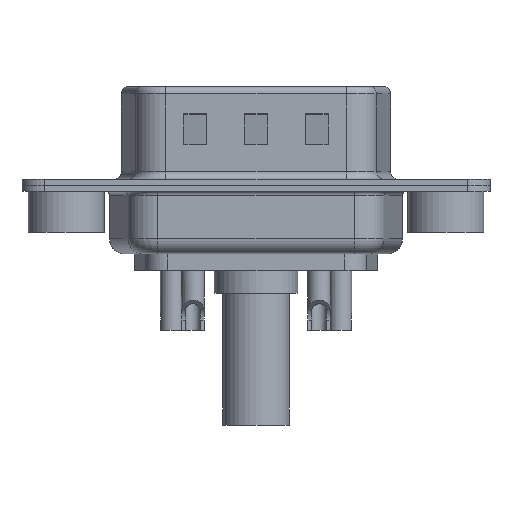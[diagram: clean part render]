
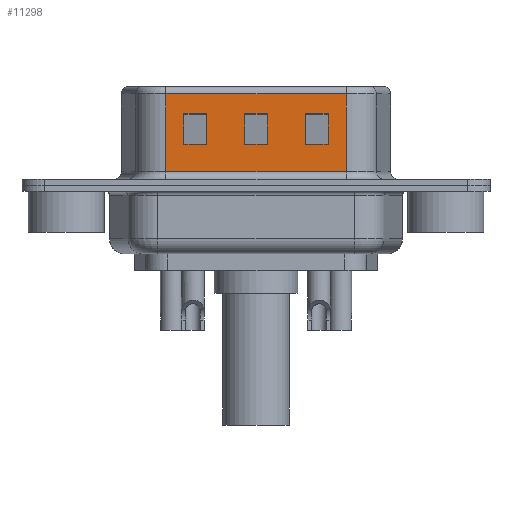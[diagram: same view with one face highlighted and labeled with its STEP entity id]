
A CAD part, front view. The second image highlights one B-rep face of the part: STEP entity #11298.
In plain terms, the highlighted planar face has unit normal (0, -1, 0).
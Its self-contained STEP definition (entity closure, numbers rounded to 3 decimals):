
#24 = VECTOR ( 'NONE', #2627, 1000. ) ;
#166 = DIRECTION ( 'NONE',  ( 0., 0., 1. ) ) ;
#189 = LINE ( 'NONE', #15808, #4331 ) ;
#196 = DIRECTION ( 'NONE',  ( -1., 0., 0. ) ) ;
#647 = CARTESIAN_POINT ( 'NONE',  ( 18.45, -4.58, 6.02 ) ) ;
#765 = EDGE_LOOP ( 'NONE', ( #6442, #6425, #10192, #7241 ) ) ;
#857 = EDGE_CURVE ( 'NONE', #8389, #2195, #1545, .T. ) ;
#917 = VECTOR ( 'NONE', #13307, 1000. ) ;
#921 = LINE ( 'NONE', #5313, #24 ) ;
#1360 = CARTESIAN_POINT ( 'NONE',  ( 15.75, -4.58, 2.705 ) ) ;
#1391 = ORIENTED_EDGE ( 'NONE', *, *, #1806, .T. ) ;
#1420 = LINE ( 'NONE', #13217, #4685 ) ;
#1493 = VECTOR ( 'NONE', #16362, 1000. ) ;
#1545 = LINE ( 'NONE', #11273, #8769 ) ;
#1702 = ORIENTED_EDGE ( 'NONE', *, *, #4582, .T. ) ;
#1806 = EDGE_CURVE ( 'NONE', #4590, #8389, #2220, .T. ) ;
#1848 = VERTEX_POINT ( 'NONE', #1360 ) ;
#1966 = CARTESIAN_POINT ( 'NONE',  ( 7.75, -4.58, 4.705 ) ) ;
#2132 = ORIENTED_EDGE ( 'NONE', *, *, #857, .T. ) ;
#2195 = VERTEX_POINT ( 'NONE', #5298 ) ;
#2220 = LINE ( 'NONE', #15970, #5825 ) ;
#2395 = ORIENTED_EDGE ( 'NONE', *, *, #9380, .T. ) ;
#2528 = DIRECTION ( 'NONE',  ( 0., 0., -1. ) ) ;
#2570 = ORIENTED_EDGE ( 'NONE', *, *, #5812, .T. ) ;
#2623 = LINE ( 'NONE', #16500, #16388 ) ;
#2627 = DIRECTION ( 'NONE',  ( -1., 0., 0. ) ) ;
#2742 = EDGE_CURVE ( 'NONE', #15333, #4590, #13022, .T. ) ;
#2941 = CARTESIAN_POINT ( 'NONE',  ( 18.45, -4.58, 6.52 ) ) ;
#3029 = VERTEX_POINT ( 'NONE', #647 ) ;
#3149 = EDGE_LOOP ( 'NONE', ( #13608, #2395, #9383, #2570 ) ) ;
#3228 = DIRECTION ( 'NONE',  ( -1., 0., 0. ) ) ;
#3500 = CARTESIAN_POINT ( 'NONE',  ( 14.45, -4.58, 2.705 ) ) ;
#3504 = DIRECTION ( 'NONE',  ( 0., 0., -1. ) ) ;
#3507 = VERTEX_POINT ( 'NONE', #7086 ) ;
#3559 = LINE ( 'NONE', #10552, #7119 ) ;
#3588 = VERTEX_POINT ( 'NONE', #13491 ) ;
#3820 = CARTESIAN_POINT ( 'NONE',  ( 9.25, -4.58, 2.705 ) ) ;
#3976 = DIRECTION ( 'NONE',  ( 1., 0., 0. ) ) ;
#4067 = DIRECTION ( 'NONE',  ( 0., 0., -1. ) ) ;
#4071 = DIRECTION ( 'NONE',  ( 0., 0., 1. ) ) ;
#4331 = VECTOR ( 'NONE', #16017, 1000. ) ;
#4582 = EDGE_CURVE ( 'NONE', #2195, #15333, #6016, .T. ) ;
#4590 = VERTEX_POINT ( 'NONE', #11797 ) ;
#4685 = VECTOR ( 'NONE', #3976, 1000. ) ;
#4841 = CARTESIAN_POINT ( 'NONE',  ( 17.25, -4.58, 2.705 ) ) ;
#4879 = CARTESIAN_POINT ( 'NONE',  ( 6.55, -4.58, 6.52 ) ) ;
#4881 = ORIENTED_EDGE ( 'NONE', *, *, #17098, .T. ) ;
#4919 = EDGE_CURVE ( 'NONE', #13281, #14281, #2623, .T. ) ;
#5298 = CARTESIAN_POINT ( 'NONE',  ( 9.25, -4.58, 4.705 ) ) ;
#5313 = CARTESIAN_POINT ( 'NONE',  ( 22.45, -4.58, 2.705 ) ) ;
#5441 = CARTESIAN_POINT ( 'NONE',  ( 18.45, -4.58, 4.705 ) ) ;
#5642 = CARTESIAN_POINT ( 'NONE',  ( 18.45, -4.58, 0.9 ) ) ;
#5812 = EDGE_CURVE ( 'NONE', #3507, #8795, #189, .T. ) ;
#5825 = VECTOR ( 'NONE', #12913, 1000. ) ;
#6016 = LINE ( 'NONE', #12508, #13404 ) ;
#6020 = LINE ( 'NONE', #7359, #12657 ) ;
#6072 = FACE_BOUND ( 'NONE', #15470, .T. ) ;
#6241 = ORIENTED_EDGE ( 'NONE', *, *, #13717, .T. ) ;
#6324 = ORIENTED_EDGE ( 'NONE', *, *, #15402, .T. ) ;
#6345 = EDGE_CURVE ( 'NONE', #3029, #16842, #8722, .T. ) ;
#6425 = ORIENTED_EDGE ( 'NONE', *, *, #6345, .T. ) ;
#6442 = ORIENTED_EDGE ( 'NONE', *, *, #9281, .F. ) ;
#6564 = CARTESIAN_POINT ( 'NONE',  ( 11.75, -4.58, 4.705 ) ) ;
#6698 = CARTESIAN_POINT ( 'NONE',  ( 13.25, -4.58, 6.52 ) ) ;
#7086 = CARTESIAN_POINT ( 'NONE',  ( 11.75, -4.58, 2.705 ) ) ;
#7119 = VECTOR ( 'NONE', #2528, 1000. ) ;
#7241 = ORIENTED_EDGE ( 'NONE', *, *, #4919, .T. ) ;
#7256 = EDGE_CURVE ( 'NONE', #16842, #13281, #9732, .T. ) ;
#7359 = CARTESIAN_POINT ( 'NONE',  ( 17.25, -4.58, 6.52 ) ) ;
#7756 = LINE ( 'NONE', #5441, #917 ) ;
#8287 = VERTEX_POINT ( 'NONE', #16213 ) ;
#8330 = DIRECTION ( 'NONE',  ( 0., 1., 0. ) ) ;
#8389 = VERTEX_POINT ( 'NONE', #1966 ) ;
#8472 = VERTEX_POINT ( 'NONE', #4841 ) ;
#8491 = EDGE_CURVE ( 'NONE', #8287, #3507, #8838, .T. ) ;
#8584 = VERTEX_POINT ( 'NONE', #13718 ) ;
#8722 = LINE ( 'NONE', #11275, #1493 ) ;
#8769 = VECTOR ( 'NONE', #10226, 1000. ) ;
#8795 = VERTEX_POINT ( 'NONE', #6564 ) ;
#8838 = LINE ( 'NONE', #12781, #11943 ) ;
#9019 = VECTOR ( 'NONE', #4067, 1000. ) ;
#9281 = EDGE_CURVE ( 'NONE', #3029, #14281, #3559, .T. ) ;
#9380 = EDGE_CURVE ( 'NONE', #3588, #8287, #12522, .T. ) ;
#9383 = ORIENTED_EDGE ( 'NONE', *, *, #8491, .T. ) ;
#9629 = CARTESIAN_POINT ( 'NONE',  ( 6.55, -4.58, 6.02 ) ) ;
#9732 = LINE ( 'NONE', #4879, #12814 ) ;
#9774 = EDGE_LOOP ( 'NONE', ( #1702, #13530, #1391, #2132 ) ) ;
#10192 = ORIENTED_EDGE ( 'NONE', *, *, #7256, .T. ) ;
#10226 = DIRECTION ( 'NONE',  ( 1., 0., 0. ) ) ;
#10493 = LINE ( 'NONE', #13310, #14679 ) ;
#10552 = CARTESIAN_POINT ( 'NONE',  ( 18.45, -4.58, 6.52 ) ) ;
#11089 = ORIENTED_EDGE ( 'NONE', *, *, #12042, .T. ) ;
#11169 = EDGE_CURVE ( 'NONE', #8795, #3588, #7756, .T. ) ;
#11273 = CARTESIAN_POINT ( 'NONE',  ( 14.45, -4.58, 4.705 ) ) ;
#11275 = CARTESIAN_POINT ( 'NONE',  ( 18.45, -4.58, 6.02 ) ) ;
#11298 = ADVANCED_FACE ( 'NONE', ( #16004, #6072, #13076, #12701 ), #16054, .F. ) ;
#11797 = CARTESIAN_POINT ( 'NONE',  ( 7.75, -4.58, 2.705 ) ) ;
#11943 = VECTOR ( 'NONE', #196, 1000. ) ;
#11976 = DIRECTION ( 'NONE',  ( 1., 0., 0. ) ) ;
#12042 = EDGE_CURVE ( 'NONE', #8584, #15512, #1420, .T. ) ;
#12062 = AXIS2_PLACEMENT_3D ( 'NONE', #2941, #8330, #166 ) ;
#12508 = CARTESIAN_POINT ( 'NONE',  ( 9.25, -4.58, 6.52 ) ) ;
#12522 = LINE ( 'NONE', #6698, #9019 ) ;
#12588 = CARTESIAN_POINT ( 'NONE',  ( 6.55, -4.58, 0.9 ) ) ;
#12657 = VECTOR ( 'NONE', #16399, 1000. ) ;
#12701 = FACE_OUTER_BOUND ( 'NONE', #765, .T. ) ;
#12781 = CARTESIAN_POINT ( 'NONE',  ( 18.45, -4.58, 2.705 ) ) ;
#12814 = VECTOR ( 'NONE', #3504, 1000. ) ;
#12913 = DIRECTION ( 'NONE',  ( 0., 0., 1. ) ) ;
#13022 = LINE ( 'NONE', #3500, #15943 ) ;
#13076 = FACE_BOUND ( 'NONE', #3149, .T. ) ;
#13217 = CARTESIAN_POINT ( 'NONE',  ( 22.45, -4.58, 4.705 ) ) ;
#13281 = VERTEX_POINT ( 'NONE', #12588 ) ;
#13307 = DIRECTION ( 'NONE',  ( 1., 0., 0. ) ) ;
#13310 = CARTESIAN_POINT ( 'NONE',  ( 15.75, -4.58, 6.52 ) ) ;
#13404 = VECTOR ( 'NONE', #14069, 1000. ) ;
#13491 = CARTESIAN_POINT ( 'NONE',  ( 13.25, -4.58, 4.705 ) ) ;
#13530 = ORIENTED_EDGE ( 'NONE', *, *, #2742, .T. ) ;
#13608 = ORIENTED_EDGE ( 'NONE', *, *, #11169, .T. ) ;
#13717 = EDGE_CURVE ( 'NONE', #1848, #8584, #10493, .T. ) ;
#13718 = CARTESIAN_POINT ( 'NONE',  ( 15.75, -4.58, 4.705 ) ) ;
#14069 = DIRECTION ( 'NONE',  ( 0., 0., -1. ) ) ;
#14281 = VERTEX_POINT ( 'NONE', #5642 ) ;
#14679 = VECTOR ( 'NONE', #4071, 1000. ) ;
#15333 = VERTEX_POINT ( 'NONE', #3820 ) ;
#15402 = EDGE_CURVE ( 'NONE', #8472, #1848, #921, .T. ) ;
#15470 = EDGE_LOOP ( 'NONE', ( #4881, #6324, #6241, #11089 ) ) ;
#15512 = VERTEX_POINT ( 'NONE', #15919 ) ;
#15808 = CARTESIAN_POINT ( 'NONE',  ( 11.75, -4.58, 6.52 ) ) ;
#15919 = CARTESIAN_POINT ( 'NONE',  ( 17.25, -4.58, 4.705 ) ) ;
#15943 = VECTOR ( 'NONE', #3228, 1000. ) ;
#15970 = CARTESIAN_POINT ( 'NONE',  ( 7.75, -4.58, 6.52 ) ) ;
#16004 = FACE_BOUND ( 'NONE', #9774, .T. ) ;
#16017 = DIRECTION ( 'NONE',  ( 0., 0., 1. ) ) ;
#16054 = PLANE ( 'NONE',  #12062 ) ;
#16213 = CARTESIAN_POINT ( 'NONE',  ( 13.25, -4.58, 2.705 ) ) ;
#16362 = DIRECTION ( 'NONE',  ( -1., 0., 0. ) ) ;
#16388 = VECTOR ( 'NONE', #11976, 1000. ) ;
#16399 = DIRECTION ( 'NONE',  ( 0., 0., -1. ) ) ;
#16500 = CARTESIAN_POINT ( 'NONE',  ( 18.45, -4.58, 0.9 ) ) ;
#16842 = VERTEX_POINT ( 'NONE', #9629 ) ;
#17098 = EDGE_CURVE ( 'NONE', #15512, #8472, #6020, .T. ) ;
